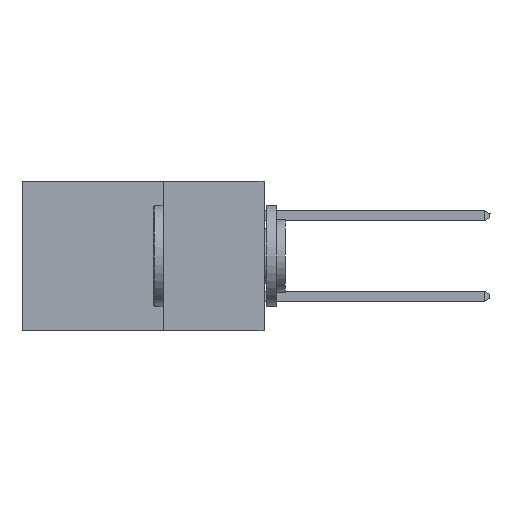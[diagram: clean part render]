
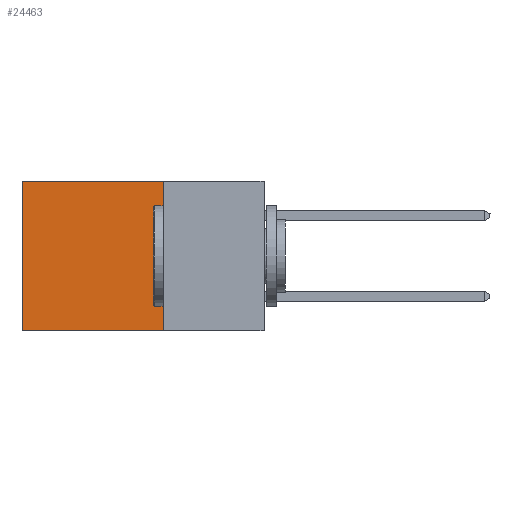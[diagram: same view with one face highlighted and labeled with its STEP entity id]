
A CAD part, left-side view. The second image highlights one B-rep face of the part: STEP entity #24463.
In plain terms, the highlighted planar face has unit normal (-1, 0, 0).
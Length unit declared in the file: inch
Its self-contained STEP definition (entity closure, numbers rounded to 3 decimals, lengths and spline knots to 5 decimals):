
#548 = VECTOR ( 'NONE', #13861, 39.37008 ) ;
#1591 = VERTEX_POINT ( 'NONE', #6356 ) ;
#2512 = DIRECTION ( 'NONE',  ( 0., 0., -1. ) ) ;
#2811 = VERTEX_POINT ( 'NONE', #15305 ) ;
#2895 = VECTOR ( 'NONE', #22892, 39.37008 ) ;
#3309 = AXIS2_PLACEMENT_3D ( 'NONE', #19145, #7964, #17305 ) ;
#4611 = CARTESIAN_POINT ( 'NONE',  ( 0.298, 0.6, 0. ) ) ;
#5116 = ORIENTED_EDGE ( 'NONE', *, *, #22215, .F. ) ;
#5390 = LINE ( 'NONE', #24798, #548 ) ;
#6283 = EDGE_CURVE ( 'NONE', #2811, #22965, #17946, .T. ) ;
#6356 = CARTESIAN_POINT ( 'NONE',  ( 0.298, 0.25, 0. ) ) ;
#7849 = ORIENTED_EDGE ( 'NONE', *, *, #24847, .T. ) ;
#7964 = DIRECTION ( 'NONE',  ( 1., 0., 0. ) ) ;
#8321 = CARTESIAN_POINT ( 'NONE',  ( 0.298, 0.25, -0.37 ) ) ;
#8779 = FACE_OUTER_BOUND ( 'NONE', #10363, .T. ) ;
#10363 = EDGE_LOOP ( 'NONE', ( #12810, #5116, #20255, #7849 ) ) ;
#10639 = LINE ( 'NONE', #16101, #2895 ) ;
#10848 = VECTOR ( 'NONE', #22996, 39.37008 ) ;
#11255 = CARTESIAN_POINT ( 'NONE',  ( 0.298, 0.25, 0. ) ) ;
#12221 = VECTOR ( 'NONE', #2512, 39.37008 ) ;
#12810 = ORIENTED_EDGE ( 'NONE', *, *, #6283, .T. ) ;
#13534 = LINE ( 'NONE', #11255, #10848 ) ;
#13861 = DIRECTION ( 'NONE',  ( 0., 0., -1. ) ) ;
#15305 = CARTESIAN_POINT ( 'NONE',  ( 0.298, 0.6, 0. ) ) ;
#16101 = CARTESIAN_POINT ( 'NONE',  ( 0.298, 0.25, -0.37 ) ) ;
#17190 = VERTEX_POINT ( 'NONE', #8321 ) ;
#17305 = DIRECTION ( 'NONE',  ( 0., 0., -1. ) ) ;
#17946 = LINE ( 'NONE', #4611, #12221 ) ;
#19145 = CARTESIAN_POINT ( 'NONE',  ( 0.298, 0.25, 0. ) ) ;
#19446 = PLANE ( 'NONE',  #3309 ) ;
#20045 = EDGE_CURVE ( 'NONE', #1591, #17190, #5390, .T. ) ;
#20255 = ORIENTED_EDGE ( 'NONE', *, *, #20045, .F. ) ;
#22215 = EDGE_CURVE ( 'NONE', #17190, #22965, #10639, .T. ) ;
#22892 = DIRECTION ( 'NONE',  ( 0., 1., 0. ) ) ;
#22965 = VERTEX_POINT ( 'NONE', #23809 ) ;
#22996 = DIRECTION ( 'NONE',  ( 0., 1., 0. ) ) ;
#23809 = CARTESIAN_POINT ( 'NONE',  ( 0.298, 0.6, -0.37 ) ) ;
#24463 = ADVANCED_FACE ( 'NONE', ( #8779 ), #19446, .F. ) ;
#24798 = CARTESIAN_POINT ( 'NONE',  ( 0.298, 0.25, 0. ) ) ;
#24847 = EDGE_CURVE ( 'NONE', #1591, #2811, #13534, .T. ) ;
